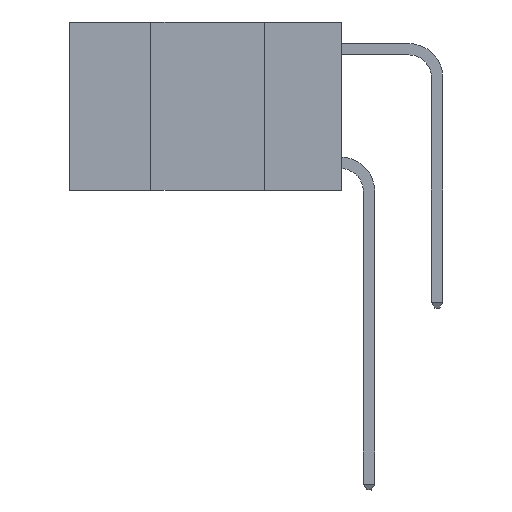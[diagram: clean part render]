
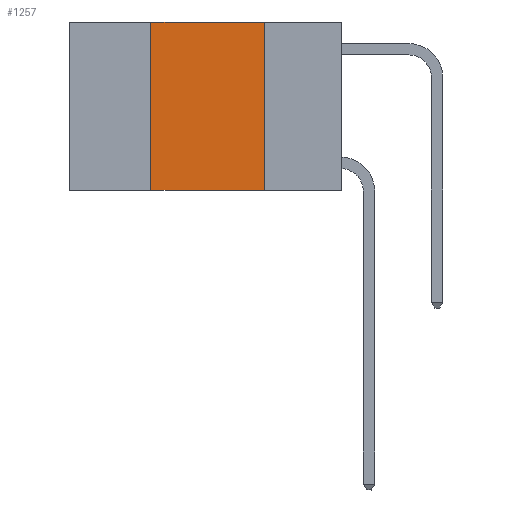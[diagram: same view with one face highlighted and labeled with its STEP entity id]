
A CAD part, left-side view. The second image highlights one B-rep face of the part: STEP entity #1257.
In plain terms, the highlighted planar face has unit normal (-1, 0, 0).
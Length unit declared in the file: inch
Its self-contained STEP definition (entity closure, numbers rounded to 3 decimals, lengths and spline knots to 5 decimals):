
#980 = LINE ( 'NONE', #29042, #13899 ) ;
#1257 = ADVANCED_FACE ( 'NONE', ( #7833 ), #3709, .F. ) ;
#1807 = CARTESIAN_POINT ( 'NONE',  ( 0., 0.42, -0.37 ) ) ;
#2104 = EDGE_CURVE ( 'NONE', #5703, #9809, #28942, .T. ) ;
#2638 = LINE ( 'NONE', #21836, #17008 ) ;
#2738 = DIRECTION ( 'NONE',  ( 0., 0., -1. ) ) ;
#3709 = PLANE ( 'NONE',  #26455 ) ;
#4534 = CARTESIAN_POINT ( 'NONE',  ( 0., 0.17, -0.37 ) ) ;
#5703 = VERTEX_POINT ( 'NONE', #15668 ) ;
#6332 = CARTESIAN_POINT ( 'NONE',  ( 0., 0.17, 0. ) ) ;
#7833 = FACE_OUTER_BOUND ( 'NONE', #23034, .T. ) ;
#7894 = ORIENTED_EDGE ( 'NONE', *, *, #23546, .F. ) ;
#9028 = DIRECTION ( 'NONE',  ( 0., -1., 0. ) ) ;
#9809 = VERTEX_POINT ( 'NONE', #4534 ) ;
#10527 = VERTEX_POINT ( 'NONE', #21593 ) ;
#10982 = VECTOR ( 'NONE', #9028, 39.37008 ) ;
#12008 = EDGE_CURVE ( 'NONE', #29811, #9809, #2638, .T. ) ;
#12518 = DIRECTION ( 'NONE',  ( 0., 0., 1. ) ) ;
#13554 = ORIENTED_EDGE ( 'NONE', *, *, #2104, .F. ) ;
#13899 = VECTOR ( 'NONE', #12518, 39.37008 ) ;
#15087 = EDGE_CURVE ( 'NONE', #10527, #5703, #29863, .T. ) ;
#15277 = DIRECTION ( 'NONE',  ( 1., 0., 0. ) ) ;
#15668 = CARTESIAN_POINT ( 'NONE',  ( 0., 0.17, 0. ) ) ;
#17008 = VECTOR ( 'NONE', #26491, 39.37008 ) ;
#18513 = CARTESIAN_POINT ( 'NONE',  ( 0., 0.6, 0. ) ) ;
#21593 = CARTESIAN_POINT ( 'NONE',  ( 0., 0.42, 0. ) ) ;
#21836 = CARTESIAN_POINT ( 'NONE',  ( 0., 0.6, -0.37 ) ) ;
#22549 = DIRECTION ( 'NONE',  ( 0., 0., -1. ) ) ;
#23034 = EDGE_LOOP ( 'NONE', ( #13554, #26106, #7894, #27598 ) ) ;
#23250 = CARTESIAN_POINT ( 'NONE',  ( 0., 0.6, 0. ) ) ;
#23546 = EDGE_CURVE ( 'NONE', #29811, #10527, #980, .T. ) ;
#26106 = ORIENTED_EDGE ( 'NONE', *, *, #15087, .F. ) ;
#26455 = AXIS2_PLACEMENT_3D ( 'NONE', #23250, #15277, #2738 ) ;
#26491 = DIRECTION ( 'NONE',  ( 0., -1., 0. ) ) ;
#27598 = ORIENTED_EDGE ( 'NONE', *, *, #12008, .T. ) ;
#28199 = VECTOR ( 'NONE', #22549, 39.37008 ) ;
#28942 = LINE ( 'NONE', #6332, #28199 ) ;
#29042 = CARTESIAN_POINT ( 'NONE',  ( 0., 0.42, 0. ) ) ;
#29811 = VERTEX_POINT ( 'NONE', #1807 ) ;
#29863 = LINE ( 'NONE', #18513, #10982 ) ;
